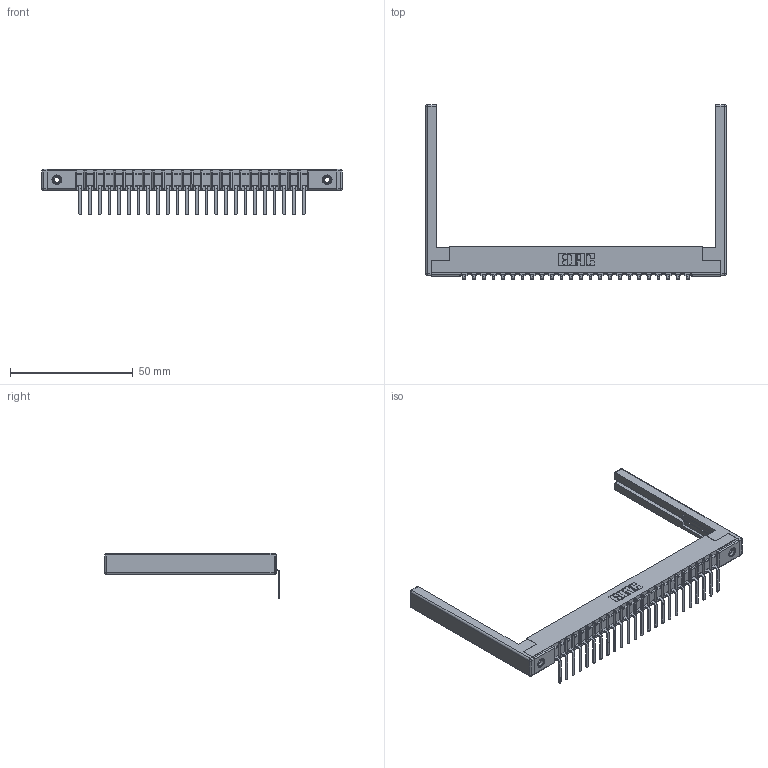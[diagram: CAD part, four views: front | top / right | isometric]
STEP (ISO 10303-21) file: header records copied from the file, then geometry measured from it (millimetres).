
FILE_DESCRIPTION (( 'STEP AP203' ), '1' );
FILE_NAME ('357-024-557-168.STEP', '2019-09-17T00:25:09', ( '' ), ( '' ), 'SwSTEP 2.0', 'SolidWorks 2016', '' );
FILE_SCHEMA (( 'CONFIG_CONTROL_DESIGN' ));
Length unit declared in the file: inch
Products named in the file (5): 307-290-002_557; 307-220-068; 345-250-001_345-250-001-102; 357-024-557-168; 307 Part_.156 Dia Mounting Holes
Assembly tree (29 placements, depth 2):
  357-024-557-168
    307 Part_.156 Dia Mounting Holes
    307-290-002_557  x24
    307-220-068  x2
    345-250-001_345-250-001-102  x2
Bounding box: 122.53 x 71.29 x 18.67 mm (x, y, z)
Volume: 12713.8 mm3; surface area: 19360.1 mm2
Topology: 29 solids, 29 shells, 2169 faces, 6569 edges, 4290 vertices
Faces by surface type: plane 1286, cylinder 809, sphere 58, cone 12, torus 4
Entity records: 26407 total; most frequent: CARTESIAN_POINT 4417, ORIENTED_EDGE 4396, DIRECTION 4318, EDGE_CURVE 2198, VECTOR 1672, LINE 1672, VERTEX_POINT 1422, AXIS2_PLACEMENT_3D 1323
